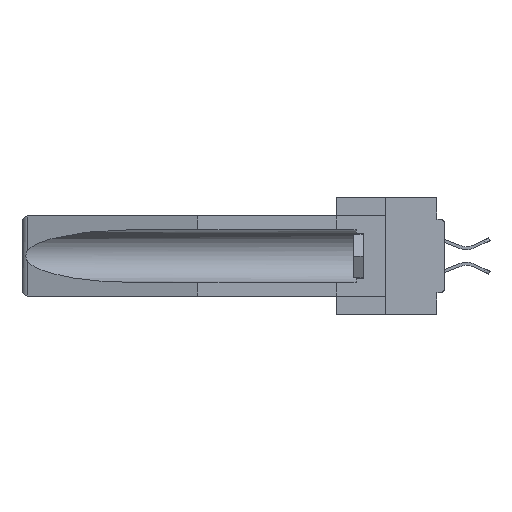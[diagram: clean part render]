
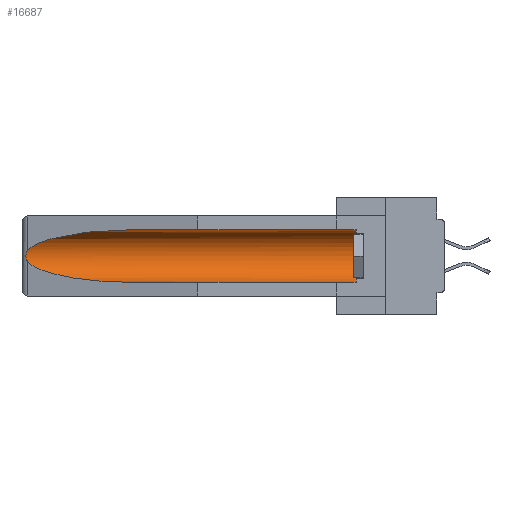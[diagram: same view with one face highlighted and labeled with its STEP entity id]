
A CAD part, left-side view. The second image highlights one B-rep face of the part: STEP entity #16687.
In plain terms, the highlighted cylindrical face has radius 2.857 mm (diameter 5.715 mm), a partial arc.
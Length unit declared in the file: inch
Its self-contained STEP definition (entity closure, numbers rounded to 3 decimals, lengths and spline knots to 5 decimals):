
#692 = ORIENTED_EDGE ( 'NONE', *, *, #33824, .T. ) ;
#1469 = CARTESIAN_POINT ( 'NONE',  ( 0.25451, 1.48313, -0.09465 ) ) ;
#1733 = LINE ( 'NONE', #20238, #5237 ) ;
#2604 = ORIENTED_EDGE ( 'NONE', *, *, #28075, .T. ) ;
#2886 = CARTESIAN_POINT ( 'NONE',  ( 0.155, 0.126, -0.059 ) ) ;
#3721 = EDGE_LOOP ( 'NONE', ( #25139, #2604, #28696, #32588, #30300, #692 ) ) ;
#4022 = CARTESIAN_POINT ( 'NONE',  ( 0.26537, 1.52718, -0.19328 ) ) ;
#4290 = CARTESIAN_POINT ( 'NONE',  ( 0.155, 0.126, -0.284 ) ) ;
#5162 = CARTESIAN_POINT ( 'NONE',  ( 0.26537, 1.52718, -0.19328 ) ) ;
#5237 = VECTOR ( 'NONE', #6166, 39.37008 ) ;
#6166 = DIRECTION ( 'NONE',  ( 0., 1., 0. ) ) ;
#6853 = EDGE_CURVE ( 'NONE', #32212, #31403, #36558, .T. ) ;
#7107 = FACE_OUTER_BOUND ( 'NONE', #3721, .T. ) ;
#8477 = VERTEX_POINT ( 'NONE', #29317 ) ;
#9503 = CARTESIAN_POINT ( 'NONE',  ( 0.26537, 1.52718, -0.14972 ) ) ;
#9876 = DIRECTION ( 'NONE',  ( 0., 1., 0. ) ) ;
#9899 = AXIS2_PLACEMENT_3D ( 'NONE', #35658, #9876, #12597 ) ;
#12218 = CARTESIAN_POINT ( 'NONE',  ( 0.2675, 1.53308, -0.16763 ) ) ;
#12298 = CARTESIAN_POINT ( 'NONE',  ( 0.26537, 1.52718, -0.14972 ) ) ;
#12597 = DIRECTION ( 'NONE',  ( 0., 0., 1. ) ) ;
#12878 = EDGE_CURVE ( 'NONE', #23104, #8477, #1733, .T. ) ;
#13128 = CARTESIAN_POINT ( 'NONE',  ( 0.155, -0.30754, -0.059 ) ) ;
#13242 = CARTESIAN_POINT ( 'NONE',  ( 0.26537, 1.52718, -0.19328 ) ) ;
#13848 = CARTESIAN_POINT ( 'NONE',  ( 0.155, 1.07973, -0.284 ) ) ;
#14524 = DIRECTION ( 'NONE',  ( 0., 0., 1. ) ) ;
#15412 = CARTESIAN_POINT ( 'NONE',  ( 0.2673, 1.53269, -0.17917 ) ) ;
#15529 = CARTESIAN_POINT ( 'NONE',  ( 0.155, 1.07973, -0.059 ) ) ;
#15726 = CARTESIAN_POINT ( 'NONE',  ( 0.155, 1.07973, -0.059 ) ) ;
#16428 = CARTESIAN_POINT ( 'NONE',  ( 0.21114, 1.30732, -0.284 ) ) ;
#16687 = ADVANCED_FACE ( 'NONE', ( #7107 ), #23003, .F. ) ;
#18356 = CARTESIAN_POINT ( 'NONE',  ( 0.26597, 1.5296, -0.19026 ) ) ;
#18947 = AXIS2_PLACEMENT_3D ( 'NONE', #23516, #34408, #14524 ) ;
#19934 = EDGE_CURVE ( 'NONE', #23104, #27519, #25392, .T. ) ;
#20238 = CARTESIAN_POINT ( 'NONE',  ( 0.155, -0.30754, -0.284 ) ) ;
#20820 = CARTESIAN_POINT ( 'NONE',  ( 0.26654, 1.53092, -0.15636 ) ) ;
#21246 = CARTESIAN_POINT ( 'NONE',  ( 0.26537, 1.52718, -0.14972 ) ) ;
#23003 = CYLINDRICAL_SURFACE ( 'NONE', #9899, 0.1125 ) ;
#23104 = VERTEX_POINT ( 'NONE', #4290 ) ;
#23425 = CARTESIAN_POINT ( 'NONE',  ( 0.26655, 1.53094, -0.18657 ) ) ;
#23516 = CARTESIAN_POINT ( 'NONE',  ( 0.155, 0.126, -0.1715 ) ) ;
#23910 = B_SPLINE_CURVE_WITH_KNOTS ( 'NONE', 3,
 ( #9503, #26776, #20820, #35294, #12218, #29234, #15412, #23425, #18356, #4022 ),
 .UNSPECIFIED., .F., .F.,
 ( 4, 2, 2, 2, 4 ),
 ( 0., 0.00029, 0.00058, 0.00087, 0.00117 ),
 .UNSPECIFIED. ) ;
#25139 = ORIENTED_EDGE ( 'NONE', *, *, #6853, .T. ) ;
#25392 = CIRCLE ( 'NONE', #18947, 0.1125 ) ;
#26079 = VECTOR ( 'NONE', #27213, 39.37008 ) ;
#26776 = CARTESIAN_POINT ( 'NONE',  ( 0.26597, 1.52961, -0.15275 ) ) ;
#27211 = VERTEX_POINT ( 'NONE', #13242 ) ;
#27213 = DIRECTION ( 'NONE',  ( 0., 1., 0. ) ) ;
#27519 = VERTEX_POINT ( 'NONE', #2886 ) ;
#28075 = EDGE_CURVE ( 'NONE', #31403, #27211, #23910, .T. ) ;
#28292 = LINE ( 'NONE', #13128, #26079 ) ;
#28696 = ORIENTED_EDGE ( 'NONE', *, *, #36394, .T. ) ;
#29234 = CARTESIAN_POINT ( 'NONE',  ( 0.2675, 1.53308, -0.17534 ) ) ;
#29317 = CARTESIAN_POINT ( 'NONE',  ( 0.155, 1.07973, -0.284 ) ) ;
#29551 = CARTESIAN_POINT ( 'NONE',  ( 0.21114, 1.30732, -0.059 ) ) ;
#30300 = ORIENTED_EDGE ( 'NONE', *, *, #19934, .T. ) ;
#31403 = VERTEX_POINT ( 'NONE', #12298 ) ;
#32212 = VERTEX_POINT ( 'NONE', #15529 ) ;
#32588 = ORIENTED_EDGE ( 'NONE', *, *, #12878, .F. ) ;
#33356 = CARTESIAN_POINT ( 'NONE',  ( 0.25451, 1.48313, -0.24835 ) ) ;
#33824 = EDGE_CURVE ( 'NONE', #27519, #32212, #28292, .T. ) ;
#34408 = DIRECTION ( 'NONE',  ( 0., -1., 0. ) ) ;
#35013 =( BOUNDED_CURVE ( )  B_SPLINE_CURVE ( 3, ( #5162, #33356, #16428, #13848 ),
 .UNSPECIFIED., .F., .F. ) 
 B_SPLINE_CURVE_WITH_KNOTS ( ( 4, 4 ),
 ( 0.1948, 1.5708 ),
 .UNSPECIFIED. ) 
 CURVE ( )  GEOMETRIC_REPRESENTATION_ITEM ( )  RATIONAL_B_SPLINE_CURVE ( ( 1., 0.848, 0.848, 1. ) ) 
 REPRESENTATION_ITEM ( '' )  );
#35294 = CARTESIAN_POINT ( 'NONE',  ( 0.2673, 1.5327, -0.16383 ) ) ;
#35658 = CARTESIAN_POINT ( 'NONE',  ( 0.155, -0.30754, -0.1715 ) ) ;
#36394 = EDGE_CURVE ( 'NONE', #27211, #8477, #35013, .T. ) ;
#36558 =( BOUNDED_CURVE ( )  B_SPLINE_CURVE ( 3, ( #15726, #29551, #1469, #21246 ),
 .UNSPECIFIED., .F., .F. ) 
 B_SPLINE_CURVE_WITH_KNOTS ( ( 4, 4 ),
 ( 4.71239, 6.08839 ),
 .UNSPECIFIED. ) 
 CURVE ( )  GEOMETRIC_REPRESENTATION_ITEM ( )  RATIONAL_B_SPLINE_CURVE ( ( 1., 0.848, 0.848, 1. ) ) 
 REPRESENTATION_ITEM ( '' )  );
